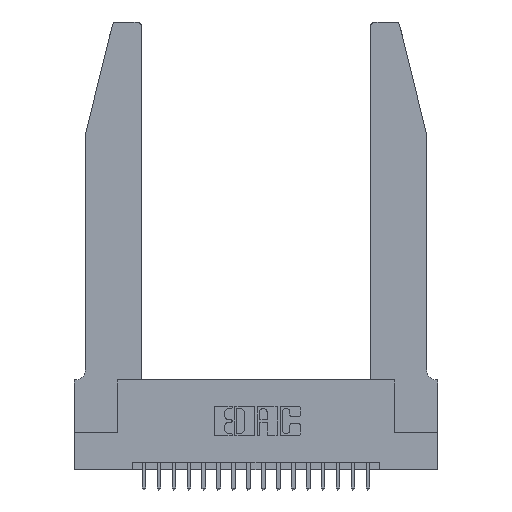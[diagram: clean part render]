
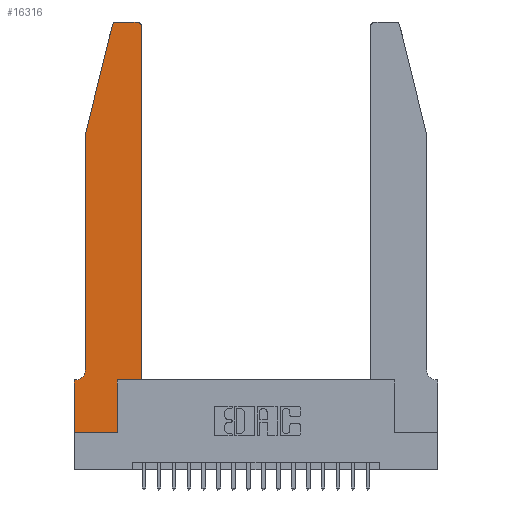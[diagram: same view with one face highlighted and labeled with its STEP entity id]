
A CAD part, top view. The second image highlights one B-rep face of the part: STEP entity #16316.
In plain terms, the highlighted planar face has unit normal (0, 0, 1).
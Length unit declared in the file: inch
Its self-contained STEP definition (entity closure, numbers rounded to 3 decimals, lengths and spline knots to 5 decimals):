
#89 = DIRECTION ( 'NONE',  ( 0., 1., 0. ) ) ;
#175 = DIRECTION ( 'NONE',  ( -0.239, -0.971, 0. ) ) ;
#306 = VECTOR ( 'NONE', #5266, 39.37008 ) ;
#580 = CIRCLE ( 'NONE', #11997, 0.03 ) ;
#612 = CARTESIAN_POINT ( 'NONE',  ( 0.284, 2.75, 0.37 ) ) ;
#788 = DIRECTION ( 'NONE',  ( 1., 0., 0. ) ) ;
#940 = ORIENTED_EDGE ( 'NONE', *, *, #15373, .T. ) ;
#1202 = LINE ( 'NONE', #1435, #5477 ) ;
#1435 = CARTESIAN_POINT ( 'NONE',  ( 0.0755, 0.35, 0.37 ) ) ;
#1629 = CARTESIAN_POINT ( 'NONE',  ( 0.4205, 2.75, 0.37 ) ) ;
#1709 = CIRCLE ( 'NONE', #11492, 0.07 ) ;
#1831 = EDGE_CURVE ( 'NONE', #12321, #20075, #1202, .T. ) ;
#1854 = VECTOR ( 'NONE', #17994, 39.37008 ) ;
#1918 = ORIENTED_EDGE ( 'NONE', *, *, #11132, .T. ) ;
#2114 = EDGE_CURVE ( 'NONE', #3708, #17357, #3715, .T. ) ;
#2161 = DIRECTION ( 'NONE',  ( 1., 0., 0. ) ) ;
#2737 = CARTESIAN_POINT ( 'NONE',  ( 0.284, 2.72, 0.37 ) ) ;
#2738 = DIRECTION ( 'NONE',  ( 0., -1., 0. ) ) ;
#2938 = EDGE_CURVE ( 'NONE', #7485, #12761, #9928, .T. ) ;
#3093 = CARTESIAN_POINT ( 'NONE',  ( 0.4505, 0.35, 0.37 ) ) ;
#3293 = VECTOR ( 'NONE', #89, 39.37008 ) ;
#3459 = CARTESIAN_POINT ( 'NONE',  ( 0.4505, 0.35, 0.37 ) ) ;
#3461 = VECTOR ( 'NONE', #2738, 39.37008 ) ;
#3535 = ORIENTED_EDGE ( 'NONE', *, *, #8251, .T. ) ;
#3708 = VERTEX_POINT ( 'NONE', #12101 ) ;
#3715 = LINE ( 'NONE', #4039, #7433 ) ;
#4039 = CARTESIAN_POINT ( 'NONE',  ( 0., 0., 0.37 ) ) ;
#4205 = VERTEX_POINT ( 'NONE', #8387 ) ;
#4370 = DIRECTION ( 'NONE',  ( 1., 0., 0. ) ) ;
#4883 = EDGE_LOOP ( 'NONE', ( #18044, #15440, #3535, #15500, #1918, #16971, #940, #17857, #9223, #8514, #20741, #6777 ) ) ;
#5081 = LINE ( 'NONE', #10021, #306 ) ;
#5097 = CARTESIAN_POINT ( 'NONE',  ( 0., 0.35, 0.37 ) ) ;
#5120 = CARTESIAN_POINT ( 'NONE',  ( 0.2865, 0.35, 0.37 ) ) ;
#5155 = EDGE_CURVE ( 'NONE', #20337, #18829, #17179, .T. ) ;
#5266 = DIRECTION ( 'NONE',  ( -1., 0., 0. ) ) ;
#5477 = VECTOR ( 'NONE', #15691, 39.37008 ) ;
#6078 = CARTESIAN_POINT ( 'NONE',  ( 0.0055, 0.42, 0.37 ) ) ;
#6177 = CARTESIAN_POINT ( 'NONE',  ( 0.4505, 0.35, 0.37 ) ) ;
#6469 = CARTESIAN_POINT ( 'NONE',  ( 0.0755, 0.42, 0.37 ) ) ;
#6777 = ORIENTED_EDGE ( 'NONE', *, *, #2938, .T. ) ;
#6877 = EDGE_CURVE ( 'NONE', #17087, #7485, #7523, .T. ) ;
#7077 = CARTESIAN_POINT ( 'NONE',  ( 0., 0.35, 0.37 ) ) ;
#7190 = LINE ( 'NONE', #12378, #3461 ) ;
#7297 = EDGE_CURVE ( 'NONE', #15793, #4205, #580, .T. ) ;
#7433 = VECTOR ( 'NONE', #12422, 39.37008 ) ;
#7485 = VERTEX_POINT ( 'NONE', #17575 ) ;
#7523 = LINE ( 'NONE', #6177, #3293 ) ;
#7667 = DIRECTION ( 'NONE',  ( -1., 0., 0. ) ) ;
#7746 = CARTESIAN_POINT ( 'NONE',  ( 0.4205, 2.72, 0.37 ) ) ;
#8040 = LINE ( 'NONE', #9779, #12871 ) ;
#8251 = EDGE_CURVE ( 'NONE', #4205, #20337, #8040, .T. ) ;
#8387 = CARTESIAN_POINT ( 'NONE',  ( 0.25487, 2.72718, 0.37 ) ) ;
#8514 = ORIENTED_EDGE ( 'NONE', *, *, #18917, .T. ) ;
#8600 = CARTESIAN_POINT ( 'NONE',  ( 0.2865, 0., 0.37 ) ) ;
#9223 = ORIENTED_EDGE ( 'NONE', *, *, #17734, .T. ) ;
#9779 = CARTESIAN_POINT ( 'NONE',  ( 0.0755, 2., 0.37 ) ) ;
#9928 = CIRCLE ( 'NONE', #11814, 0.03 ) ;
#10021 = CARTESIAN_POINT ( 'NONE',  ( 0.2605, 2.75, 0.37 ) ) ;
#10147 = CARTESIAN_POINT ( 'NONE',  ( 0.0055, 0.35, 0.37 ) ) ;
#10397 = LINE ( 'NONE', #5120, #1854 ) ;
#10411 = DIRECTION ( 'NONE',  ( 0., 0., 1. ) ) ;
#11132 = EDGE_CURVE ( 'NONE', #18829, #12321, #1709, .T. ) ;
#11185 = DIRECTION ( 'NONE',  ( 0., 0., 1. ) ) ;
#11216 = CARTESIAN_POINT ( 'NONE',  ( 0.2865, 0.35, 0.37 ) ) ;
#11266 = VERTEX_POINT ( 'NONE', #11216 ) ;
#11492 = AXIS2_PLACEMENT_3D ( 'NONE', #6078, #17350, #7667 ) ;
#11814 = AXIS2_PLACEMENT_3D ( 'NONE', #7746, #11185, #2161 ) ;
#11997 = AXIS2_PLACEMENT_3D ( 'NONE', #2737, #14010, #4370 ) ;
#12101 = CARTESIAN_POINT ( 'NONE',  ( 0., 0., 0.37 ) ) ;
#12130 = LINE ( 'NONE', #3459, #15705 ) ;
#12321 = VERTEX_POINT ( 'NONE', #10147 ) ;
#12378 = CARTESIAN_POINT ( 'NONE',  ( 0., 0., 0.37 ) ) ;
#12422 = DIRECTION ( 'NONE',  ( 1., 0., 0. ) ) ;
#12761 = VERTEX_POINT ( 'NONE', #1629 ) ;
#12871 = VECTOR ( 'NONE', #175, 39.37008 ) ;
#12893 = CARTESIAN_POINT ( 'NONE',  ( 0.0755, 2., 0.37 ) ) ;
#12896 = VECTOR ( 'NONE', #16122, 39.37008 ) ;
#14010 = DIRECTION ( 'NONE',  ( 0., 0., 1. ) ) ;
#15373 = EDGE_CURVE ( 'NONE', #20075, #3708, #7190, .T. ) ;
#15440 = ORIENTED_EDGE ( 'NONE', *, *, #7297, .T. ) ;
#15500 = ORIENTED_EDGE ( 'NONE', *, *, #5155, .T. ) ;
#15691 = DIRECTION ( 'NONE',  ( -1., 0., 0. ) ) ;
#15705 = VECTOR ( 'NONE', #19521, 39.37008 ) ;
#15793 = VERTEX_POINT ( 'NONE', #612 ) ;
#16122 = DIRECTION ( 'NONE',  ( 0., -1., 0. ) ) ;
#16316 = ADVANCED_FACE ( 'NONE', ( #18019 ), #20079, .T. ) ;
#16971 = ORIENTED_EDGE ( 'NONE', *, *, #1831, .T. ) ;
#17087 = VERTEX_POINT ( 'NONE', #3093 ) ;
#17179 = LINE ( 'NONE', #12893, #12896 ) ;
#17314 = AXIS2_PLACEMENT_3D ( 'NONE', #7077, #10411, #788 ) ;
#17350 = DIRECTION ( 'NONE',  ( 0., 0., -1. ) ) ;
#17357 = VERTEX_POINT ( 'NONE', #8600 ) ;
#17575 = CARTESIAN_POINT ( 'NONE',  ( 0.4505, 2.72, 0.37 ) ) ;
#17734 = EDGE_CURVE ( 'NONE', #17357, #11266, #10397, .T. ) ;
#17857 = ORIENTED_EDGE ( 'NONE', *, *, #2114, .T. ) ;
#17994 = DIRECTION ( 'NONE',  ( 0., 1., 0. ) ) ;
#18019 = FACE_OUTER_BOUND ( 'NONE', #4883, .T. ) ;
#18044 = ORIENTED_EDGE ( 'NONE', *, *, #19525, .T. ) ;
#18604 = CARTESIAN_POINT ( 'NONE',  ( 0.0755, 2., 0.37 ) ) ;
#18829 = VERTEX_POINT ( 'NONE', #6469 ) ;
#18917 = EDGE_CURVE ( 'NONE', #11266, #17087, #12130, .T. ) ;
#19521 = DIRECTION ( 'NONE',  ( 1., 0., 0. ) ) ;
#19525 = EDGE_CURVE ( 'NONE', #12761, #15793, #5081, .T. ) ;
#20075 = VERTEX_POINT ( 'NONE', #5097 ) ;
#20079 = PLANE ( 'NONE',  #17314 ) ;
#20337 = VERTEX_POINT ( 'NONE', #18604 ) ;
#20741 = ORIENTED_EDGE ( 'NONE', *, *, #6877, .T. ) ;
